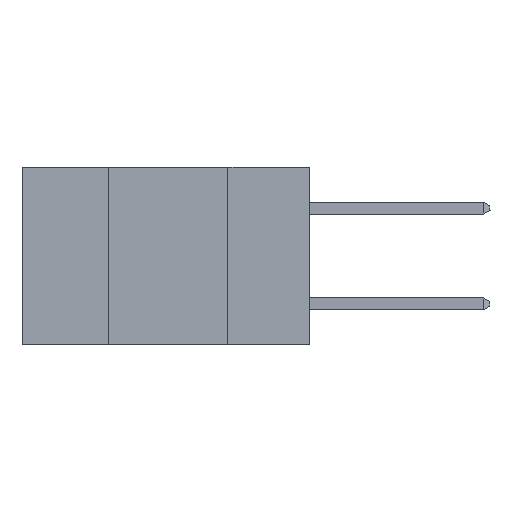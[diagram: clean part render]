
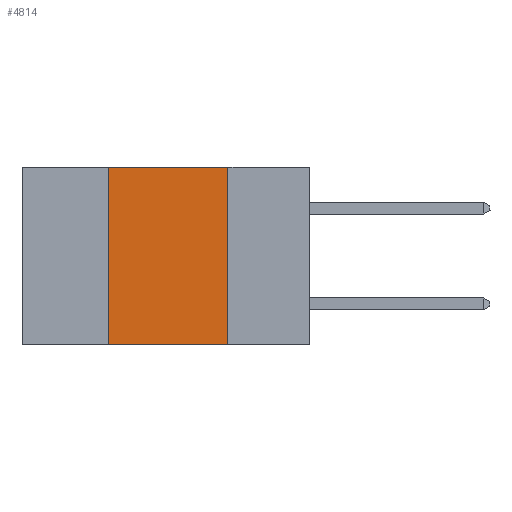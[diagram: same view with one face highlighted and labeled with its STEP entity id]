
A CAD part, left-side view. The second image highlights one B-rep face of the part: STEP entity #4814.
In plain terms, the highlighted planar face has unit normal (-1, 0, 0).
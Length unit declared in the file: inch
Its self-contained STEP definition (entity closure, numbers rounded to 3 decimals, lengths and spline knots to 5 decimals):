
#382 = CARTESIAN_POINT ( 'NONE',  ( 0., 0.6, 0. ) ) ;
#1493 = LINE ( 'NONE', #382, #11348 ) ;
#1636 = VERTEX_POINT ( 'NONE', #37454 ) ;
#4803 = VECTOR ( 'NONE', #25364, 39.37008 ) ;
#4814 = ADVANCED_FACE ( 'NONE', ( #38170 ), #32577, .F. ) ;
#5442 = DIRECTION ( 'NONE',  ( 1., 0., 0. ) ) ;
#7161 = EDGE_LOOP ( 'NONE', ( #26258, #28907, #29953, #13275 ) ) ;
#10574 = VERTEX_POINT ( 'NONE', #19383 ) ;
#10775 = CARTESIAN_POINT ( 'NONE',  ( 0., 0.6, -0.37 ) ) ;
#11007 = CARTESIAN_POINT ( 'NONE',  ( 0., 0.17, -0.37 ) ) ;
#11050 = VERTEX_POINT ( 'NONE', #34104 ) ;
#11348 = VECTOR ( 'NONE', #27704, 39.37008 ) ;
#11428 = DIRECTION ( 'NONE',  ( 0., 0., -1. ) ) ;
#12573 = AXIS2_PLACEMENT_3D ( 'NONE', #38551, #5442, #11428 ) ;
#13123 = EDGE_CURVE ( 'NONE', #1636, #28091, #13210, .T. ) ;
#13210 = LINE ( 'NONE', #18592, #4803 ) ;
#13275 = ORIENTED_EDGE ( 'NONE', *, *, #38809, .T. ) ;
#15916 = EDGE_CURVE ( 'NONE', #11050, #10574, #19251, .T. ) ;
#16767 = DIRECTION ( 'NONE',  ( 0., -1., 0. ) ) ;
#18021 = EDGE_CURVE ( 'NONE', #10574, #1636, #1493, .T. ) ;
#18592 = CARTESIAN_POINT ( 'NONE',  ( 0., 0.17, 0. ) ) ;
#19251 = LINE ( 'NONE', #31817, #26481 ) ;
#19383 = CARTESIAN_POINT ( 'NONE',  ( 0., 0.42, 0. ) ) ;
#22629 = DIRECTION ( 'NONE',  ( 0., 0., 1. ) ) ;
#22860 = VECTOR ( 'NONE', #16767, 39.37008 ) ;
#25364 = DIRECTION ( 'NONE',  ( 0., 0., -1. ) ) ;
#26258 = ORIENTED_EDGE ( 'NONE', *, *, #13123, .F. ) ;
#26481 = VECTOR ( 'NONE', #22629, 39.37008 ) ;
#27704 = DIRECTION ( 'NONE',  ( 0., -1., 0. ) ) ;
#28091 = VERTEX_POINT ( 'NONE', #11007 ) ;
#28907 = ORIENTED_EDGE ( 'NONE', *, *, #18021, .F. ) ;
#29953 = ORIENTED_EDGE ( 'NONE', *, *, #15916, .F. ) ;
#31817 = CARTESIAN_POINT ( 'NONE',  ( 0., 0.42, 0. ) ) ;
#32577 = PLANE ( 'NONE',  #12573 ) ;
#34104 = CARTESIAN_POINT ( 'NONE',  ( 0., 0.42, -0.37 ) ) ;
#37454 = CARTESIAN_POINT ( 'NONE',  ( 0., 0.17, 0. ) ) ;
#38170 = FACE_OUTER_BOUND ( 'NONE', #7161, .T. ) ;
#38551 = CARTESIAN_POINT ( 'NONE',  ( 0., 0.6, 0. ) ) ;
#38809 = EDGE_CURVE ( 'NONE', #11050, #28091, #38885, .T. ) ;
#38885 = LINE ( 'NONE', #10775, #22860 ) ;
